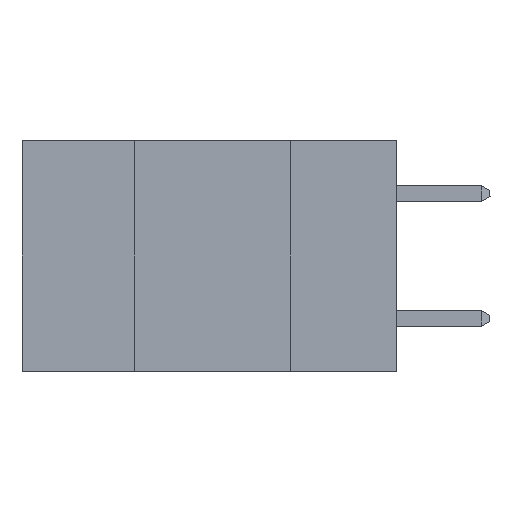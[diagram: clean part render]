
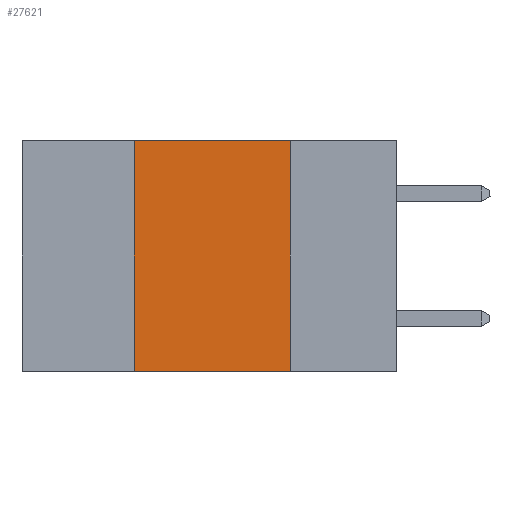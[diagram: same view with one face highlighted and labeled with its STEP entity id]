
A CAD part, left-side view. The second image highlights one B-rep face of the part: STEP entity #27621.
In plain terms, the highlighted planar face has unit normal (-1, 0, 0).
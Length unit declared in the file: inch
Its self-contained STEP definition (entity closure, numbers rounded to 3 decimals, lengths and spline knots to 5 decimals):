
#1206 = CARTESIAN_POINT ( 'NONE',  ( 0., 0.42, 0. ) ) ;
#1331 = DIRECTION ( 'NONE',  ( 0., 0., -1. ) ) ;
#2608 = CARTESIAN_POINT ( 'NONE',  ( 0., 0.6, 0. ) ) ;
#3523 = CARTESIAN_POINT ( 'NONE',  ( 0., 0.42, -0.37 ) ) ;
#3926 = EDGE_CURVE ( 'NONE', #19651, #19696, #27999, .T. ) ;
#4021 = ORIENTED_EDGE ( 'NONE', *, *, #6109, .F. ) ;
#4372 = CARTESIAN_POINT ( 'NONE',  ( 0., 0.6, 0. ) ) ;
#4569 = DIRECTION ( 'NONE',  ( 1., 0., 0. ) ) ;
#4624 = DIRECTION ( 'NONE',  ( 0., -1., 0. ) ) ;
#5392 = VECTOR ( 'NONE', #4624, 39.37008 ) ;
#6109 = EDGE_CURVE ( 'NONE', #27720, #19651, #11417, .T. ) ;
#6925 = VECTOR ( 'NONE', #19317, 39.37008 ) ;
#8711 = CARTESIAN_POINT ( 'NONE',  ( 0., 0.17, -0.37 ) ) ;
#9754 = LINE ( 'NONE', #1206, #6925 ) ;
#9891 = CARTESIAN_POINT ( 'NONE',  ( 0., 0.6, -0.37 ) ) ;
#11417 = LINE ( 'NONE', #2608, #5392 ) ;
#11822 = ORIENTED_EDGE ( 'NONE', *, *, #25984, .F. ) ;
#13555 = DIRECTION ( 'NONE',  ( 0., 0., -1. ) ) ;
#14015 = EDGE_CURVE ( 'NONE', #25432, #19696, #22122, .T. ) ;
#18066 = CARTESIAN_POINT ( 'NONE',  ( 0., 0.42, 0. ) ) ;
#18695 = ORIENTED_EDGE ( 'NONE', *, *, #3926, .F. ) ;
#18931 = VECTOR ( 'NONE', #25870, 39.37008 ) ;
#19269 = CARTESIAN_POINT ( 'NONE',  ( 0., 0.17, 0. ) ) ;
#19317 = DIRECTION ( 'NONE',  ( 0., 0., 1. ) ) ;
#19651 = VERTEX_POINT ( 'NONE', #19269 ) ;
#19696 = VERTEX_POINT ( 'NONE', #8711 ) ;
#20158 = AXIS2_PLACEMENT_3D ( 'NONE', #4372, #4569, #13555 ) ;
#21092 = ORIENTED_EDGE ( 'NONE', *, *, #14015, .T. ) ;
#22122 = LINE ( 'NONE', #9891, #18931 ) ;
#22643 = VECTOR ( 'NONE', #1331, 39.37008 ) ;
#22707 = PLANE ( 'NONE',  #20158 ) ;
#24175 = CARTESIAN_POINT ( 'NONE',  ( 0., 0.17, 0. ) ) ;
#25002 = FACE_OUTER_BOUND ( 'NONE', #29489, .T. ) ;
#25432 = VERTEX_POINT ( 'NONE', #3523 ) ;
#25870 = DIRECTION ( 'NONE',  ( 0., -1., 0. ) ) ;
#25984 = EDGE_CURVE ( 'NONE', #25432, #27720, #9754, .T. ) ;
#27621 = ADVANCED_FACE ( 'NONE', ( #25002 ), #22707, .F. ) ;
#27720 = VERTEX_POINT ( 'NONE', #18066 ) ;
#27999 = LINE ( 'NONE', #24175, #22643 ) ;
#29489 = EDGE_LOOP ( 'NONE', ( #18695, #4021, #11822, #21092 ) ) ;
